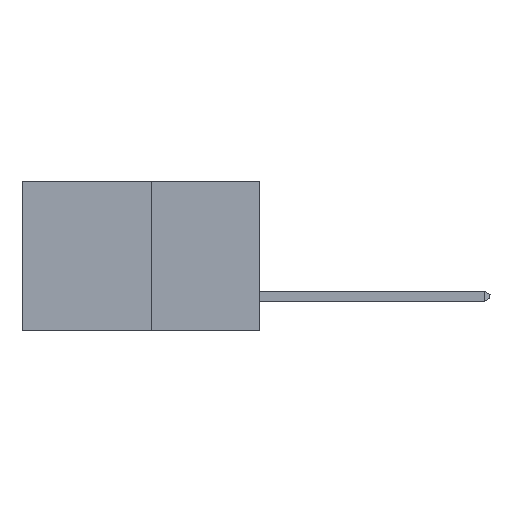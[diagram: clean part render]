
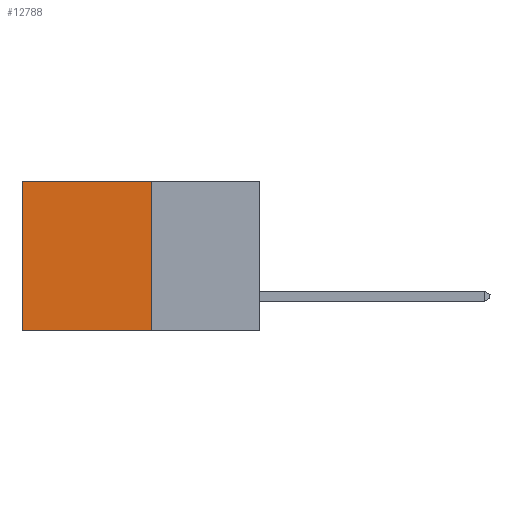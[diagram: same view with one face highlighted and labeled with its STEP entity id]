
A CAD part, left-side view. The second image highlights one B-rep face of the part: STEP entity #12788.
In plain terms, the highlighted planar face has unit normal (-1, 0, 0).
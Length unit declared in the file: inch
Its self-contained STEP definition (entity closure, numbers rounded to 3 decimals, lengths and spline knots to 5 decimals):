
#18 = VERTEX_POINT ( 'NONE', #3698 ) ;
#183 = ORIENTED_EDGE ( 'NONE', *, *, #5164, .F. ) ;
#660 = DIRECTION ( 'NONE',  ( 1., 0., 0. ) ) ;
#1748 = ORIENTED_EDGE ( 'NONE', *, *, #4293, .F. ) ;
#2003 = CARTESIAN_POINT ( 'NONE',  ( 0.277, 0.27, -0.37 ) ) ;
#2284 = ORIENTED_EDGE ( 'NONE', *, *, #7831, .T. ) ;
#2844 = DIRECTION ( 'NONE',  ( 0., 1., 0. ) ) ;
#3110 = DIRECTION ( 'NONE',  ( 0., 0., -1. ) ) ;
#3188 = LINE ( 'NONE', #12052, #8682 ) ;
#3571 = CARTESIAN_POINT ( 'NONE',  ( 0.277, 0.59, 0. ) ) ;
#3627 = LINE ( 'NONE', #10522, #6192 ) ;
#3698 = CARTESIAN_POINT ( 'NONE',  ( 0.277, 0.27, -0.37 ) ) ;
#4204 = LINE ( 'NONE', #2003, #9661 ) ;
#4293 = EDGE_CURVE ( 'NONE', #18, #7406, #3188, .T. ) ;
#5006 = VECTOR ( 'NONE', #2844, 39.37008 ) ;
#5063 = PLANE ( 'NONE',  #12414 ) ;
#5164 = EDGE_CURVE ( 'NONE', #11124, #18, #4204, .T. ) ;
#6029 = CARTESIAN_POINT ( 'NONE',  ( 0.277, 0.27, 0. ) ) ;
#6192 = VECTOR ( 'NONE', #6328, 39.37008 ) ;
#6328 = DIRECTION ( 'NONE',  ( 0., 0., -1. ) ) ;
#7406 = VERTEX_POINT ( 'NONE', #10578 ) ;
#7731 = EDGE_CURVE ( 'NONE', #11124, #8273, #7909, .T. ) ;
#7831 = EDGE_CURVE ( 'NONE', #8273, #7406, #3627, .T. ) ;
#7909 = LINE ( 'NONE', #12146, #5006 ) ;
#8273 = VERTEX_POINT ( 'NONE', #3571 ) ;
#8365 = DIRECTION ( 'NONE',  ( 0., 0., -1. ) ) ;
#8682 = VECTOR ( 'NONE', #11537, 39.37008 ) ;
#8856 = FACE_OUTER_BOUND ( 'NONE', #11244, .T. ) ;
#9661 = VECTOR ( 'NONE', #3110, 39.37008 ) ;
#10370 = CARTESIAN_POINT ( 'NONE',  ( 0.277, 0.27, -0.37 ) ) ;
#10522 = CARTESIAN_POINT ( 'NONE',  ( 0.277, 0.59, -0.37 ) ) ;
#10578 = CARTESIAN_POINT ( 'NONE',  ( 0.277, 0.59, -0.37 ) ) ;
#11124 = VERTEX_POINT ( 'NONE', #6029 ) ;
#11244 = EDGE_LOOP ( 'NONE', ( #2284, #1748, #183, #12189 ) ) ;
#11537 = DIRECTION ( 'NONE',  ( 0., 1., 0. ) ) ;
#12052 = CARTESIAN_POINT ( 'NONE',  ( 0.277, 0.27, -0.37 ) ) ;
#12146 = CARTESIAN_POINT ( 'NONE',  ( 0.277, 0.27, 0. ) ) ;
#12189 = ORIENTED_EDGE ( 'NONE', *, *, #7731, .T. ) ;
#12414 = AXIS2_PLACEMENT_3D ( 'NONE', #10370, #660, #8365 ) ;
#12788 = ADVANCED_FACE ( 'NONE', ( #8856 ), #5063, .F. ) ;
